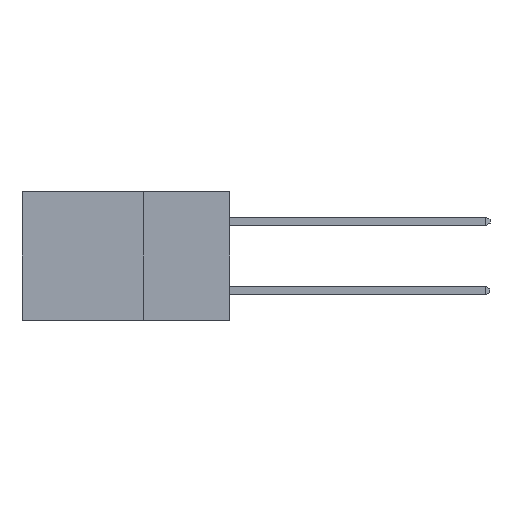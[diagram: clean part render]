
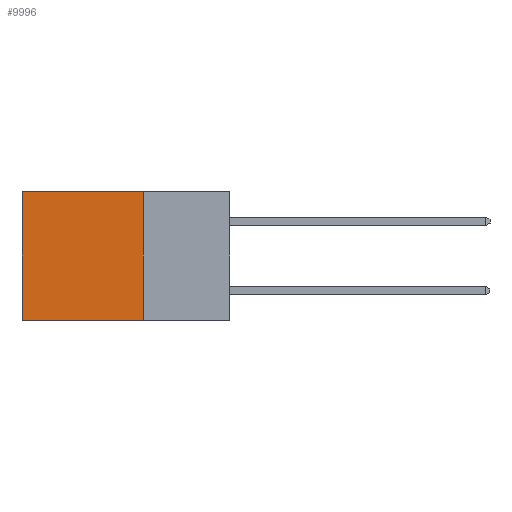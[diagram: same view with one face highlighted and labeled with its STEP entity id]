
A CAD part, left-side view. The second image highlights one B-rep face of the part: STEP entity #9996.
In plain terms, the highlighted planar face has unit normal (-1, 0, 0).
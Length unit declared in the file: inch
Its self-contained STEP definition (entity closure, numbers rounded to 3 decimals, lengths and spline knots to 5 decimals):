
#9 = CARTESIAN_POINT ( 'NONE',  ( 0.298, 0.25, 0. ) ) ;
#103 = VERTEX_POINT ( 'NONE', #13953 ) ;
#323 = ORIENTED_EDGE ( 'NONE', *, *, #9448, .F. ) ;
#728 = ORIENTED_EDGE ( 'NONE', *, *, #5298, .T. ) ;
#1098 = LINE ( 'NONE', #5600, #12230 ) ;
#1115 = DIRECTION ( 'NONE',  ( 0., 0., -1. ) ) ;
#1125 = DIRECTION ( 'NONE',  ( 1., 0., 0. ) ) ;
#1362 = LINE ( 'NONE', #5290, #9908 ) ;
#1454 = CARTESIAN_POINT ( 'NONE',  ( 0.298, 0.25, 0. ) ) ;
#1713 = ORIENTED_EDGE ( 'NONE', *, *, #11616, .F. ) ;
#1811 = FACE_OUTER_BOUND ( 'NONE', #5738, .T. ) ;
#1929 = CARTESIAN_POINT ( 'NONE',  ( 0.298, 0.6, 0. ) ) ;
#2596 = DIRECTION ( 'NONE',  ( 0., 1., 0. ) ) ;
#3732 = ORIENTED_EDGE ( 'NONE', *, *, #11843, .T. ) ;
#3944 = VERTEX_POINT ( 'NONE', #1929 ) ;
#5290 = CARTESIAN_POINT ( 'NONE',  ( 0.298, 0.6, 0. ) ) ;
#5298 = EDGE_CURVE ( 'NONE', #3944, #103, #1362, .T. ) ;
#5600 = CARTESIAN_POINT ( 'NONE',  ( 0.298, 0.25, 0. ) ) ;
#5738 = EDGE_LOOP ( 'NONE', ( #728, #323, #1713, #3732 ) ) ;
#6230 = LINE ( 'NONE', #8045, #11740 ) ;
#6720 = PLANE ( 'NONE',  #7522 ) ;
#6936 = DIRECTION ( 'NONE',  ( 0., 1., 0. ) ) ;
#7522 = AXIS2_PLACEMENT_3D ( 'NONE', #9, #1125, #8929 ) ;
#8004 = DIRECTION ( 'NONE',  ( 0., 0., -1. ) ) ;
#8045 = CARTESIAN_POINT ( 'NONE',  ( 0.298, 0.25, -0.37 ) ) ;
#8929 = DIRECTION ( 'NONE',  ( 0., 0., -1. ) ) ;
#9288 = CARTESIAN_POINT ( 'NONE',  ( 0.298, 0.25, -0.37 ) ) ;
#9448 = EDGE_CURVE ( 'NONE', #13667, #103, #6230, .T. ) ;
#9485 = VECTOR ( 'NONE', #2596, 39.37008 ) ;
#9908 = VECTOR ( 'NONE', #8004, 39.37008 ) ;
#9996 = ADVANCED_FACE ( 'NONE', ( #1811 ), #6720, .F. ) ;
#10170 = CARTESIAN_POINT ( 'NONE',  ( 0.298, 0.25, 0. ) ) ;
#11616 = EDGE_CURVE ( 'NONE', #14220, #13667, #1098, .T. ) ;
#11740 = VECTOR ( 'NONE', #6936, 39.37008 ) ;
#11843 = EDGE_CURVE ( 'NONE', #14220, #3944, #12403, .T. ) ;
#12230 = VECTOR ( 'NONE', #1115, 39.37008 ) ;
#12403 = LINE ( 'NONE', #1454, #9485 ) ;
#13667 = VERTEX_POINT ( 'NONE', #9288 ) ;
#13953 = CARTESIAN_POINT ( 'NONE',  ( 0.298, 0.6, -0.37 ) ) ;
#14220 = VERTEX_POINT ( 'NONE', #10170 ) ;
